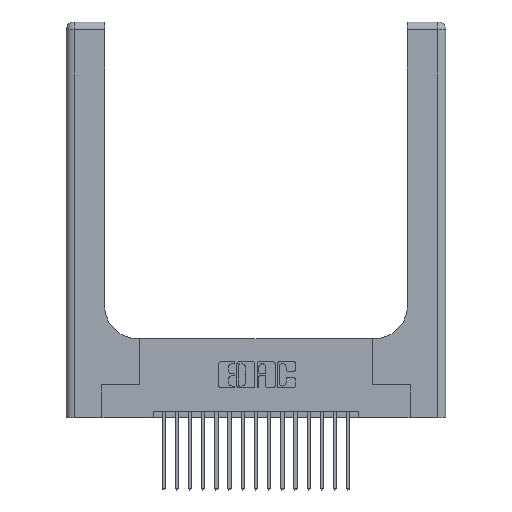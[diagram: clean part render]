
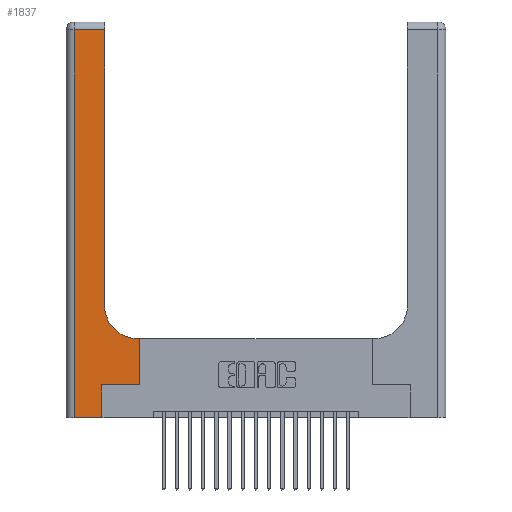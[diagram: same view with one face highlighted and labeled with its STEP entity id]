
A CAD part, top view. The second image highlights one B-rep face of the part: STEP entity #1837.
In plain terms, the highlighted planar face has unit normal (0, 0, 1).
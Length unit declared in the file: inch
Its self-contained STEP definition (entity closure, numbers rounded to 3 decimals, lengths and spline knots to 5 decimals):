
#257 = CARTESIAN_POINT ( 'NONE',  ( 0.2915, 0.85, 0.37 ) ) ;
#575 = CARTESIAN_POINT ( 'NONE',  ( 0.269, 0.25, 0.37 ) ) ;
#672 = EDGE_CURVE ( 'NONE', #4293, #8907, #10846, .T. ) ;
#947 = EDGE_CURVE ( 'NONE', #12683, #18652, #14806, .T. ) ;
#1517 = DIRECTION ( 'NONE',  ( 0., 1., 0. ) ) ;
#1659 = EDGE_CURVE ( 'NONE', #7958, #4293, #12326, .T. ) ;
#1776 = CARTESIAN_POINT ( 'NONE',  ( 0.5585, 0.25, 0.37 ) ) ;
#1837 = ADVANCED_FACE ( 'NONE', ( #2304 ), #4519, .F. ) ;
#2304 = FACE_OUTER_BOUND ( 'NONE', #10677, .T. ) ;
#2469 = CARTESIAN_POINT ( 'NONE',  ( 0.06, 2.94, 0.37 ) ) ;
#2592 = ORIENTED_EDGE ( 'NONE', *, *, #672, .T. ) ;
#2725 = AXIS2_PLACEMENT_3D ( 'NONE', #3398, #16216, #9618 ) ;
#2793 = VECTOR ( 'NONE', #1517, 39.37008 ) ;
#3398 = CARTESIAN_POINT ( 'NONE',  ( 0.5415, 0.85, 0.37 ) ) ;
#4293 = VERTEX_POINT ( 'NONE', #8136 ) ;
#4519 = PLANE ( 'NONE',  #13219 ) ;
#4549 = VECTOR ( 'NONE', #8510, 39.37008 ) ;
#4585 = DIRECTION ( 'NONE',  ( 0., 0., -1. ) ) ;
#5296 = DIRECTION ( 'NONE',  ( 1., 0., 0. ) ) ;
#5418 = LINE ( 'NONE', #10536, #17626 ) ;
#5809 = VECTOR ( 'NONE', #12511, 39.37008 ) ;
#5969 = DIRECTION ( 'NONE',  ( 0., 1., 0. ) ) ;
#6001 = VERTEX_POINT ( 'NONE', #10919 ) ;
#6007 = DIRECTION ( 'NONE',  ( -1., 0., 0. ) ) ;
#6069 = CARTESIAN_POINT ( 'NONE',  ( 0., 3., 0.37 ) ) ;
#6284 = DIRECTION ( 'NONE',  ( -1., 0., 0. ) ) ;
#6360 = ORIENTED_EDGE ( 'NONE', *, *, #1659, .T. ) ;
#6501 = ORIENTED_EDGE ( 'NONE', *, *, #14328, .T. ) ;
#7059 = EDGE_CURVE ( 'NONE', #18652, #7958, #15756, .T. ) ;
#7414 = CARTESIAN_POINT ( 'NONE',  ( 0.269, 0., 0.37 ) ) ;
#7958 = VERTEX_POINT ( 'NONE', #1776 ) ;
#8136 = CARTESIAN_POINT ( 'NONE',  ( 0.5585, 0.6, 0.37 ) ) ;
#8423 = EDGE_CURVE ( 'NONE', #6001, #12683, #16454, .T. ) ;
#8510 = DIRECTION ( 'NONE',  ( 0., 1., 0. ) ) ;
#8810 = ORIENTED_EDGE ( 'NONE', *, *, #10889, .T. ) ;
#8815 = EDGE_CURVE ( 'NONE', #9017, #10373, #9717, .T. ) ;
#8907 = VERTEX_POINT ( 'NONE', #17995 ) ;
#9017 = VERTEX_POINT ( 'NONE', #13643 ) ;
#9618 = DIRECTION ( 'NONE',  ( 1., 0., 0. ) ) ;
#9652 = ORIENTED_EDGE ( 'NONE', *, *, #8423, .T. ) ;
#9717 = LINE ( 'NONE', #11124, #15937 ) ;
#10373 = VERTEX_POINT ( 'NONE', #2469 ) ;
#10536 = CARTESIAN_POINT ( 'NONE',  ( 0.2915, 3., 0.37 ) ) ;
#10677 = EDGE_LOOP ( 'NONE', ( #12181, #19036, #6501, #9652, #14218, #12870, #6360, #2592, #8810 ) ) ;
#10846 = LINE ( 'NONE', #11133, #16059 ) ;
#10889 = EDGE_CURVE ( 'NONE', #8907, #17155, #17825, .T. ) ;
#10919 = CARTESIAN_POINT ( 'NONE',  ( 0.06, 0., 0.37 ) ) ;
#11124 = CARTESIAN_POINT ( 'NONE',  ( 0., 2.94, 0.37 ) ) ;
#11133 = CARTESIAN_POINT ( 'NONE',  ( 0.2915, 0.6, 0.37 ) ) ;
#11276 = CARTESIAN_POINT ( 'NONE',  ( 0.269, 0., 0.37 ) ) ;
#11545 = VECTOR ( 'NONE', #5296, 39.37008 ) ;
#12181 = ORIENTED_EDGE ( 'NONE', *, *, #13253, .T. ) ;
#12274 = VECTOR ( 'NONE', #16063, 39.37008 ) ;
#12326 = LINE ( 'NONE', #12909, #2793 ) ;
#12511 = DIRECTION ( 'NONE',  ( 0., -1., 0. ) ) ;
#12683 = VERTEX_POINT ( 'NONE', #7414 ) ;
#12836 = CARTESIAN_POINT ( 'NONE',  ( 0., 0., 0.37 ) ) ;
#12870 = ORIENTED_EDGE ( 'NONE', *, *, #7059, .T. ) ;
#12909 = CARTESIAN_POINT ( 'NONE',  ( 0.5585, 0.25, 0.37 ) ) ;
#13219 = AXIS2_PLACEMENT_3D ( 'NONE', #6069, #4585, #6007 ) ;
#13253 = EDGE_CURVE ( 'NONE', #17155, #9017, #5418, .T. ) ;
#13643 = CARTESIAN_POINT ( 'NONE',  ( 0.2915, 2.94, 0.37 ) ) ;
#14218 = ORIENTED_EDGE ( 'NONE', *, *, #947, .T. ) ;
#14328 = EDGE_CURVE ( 'NONE', #10373, #6001, #18724, .T. ) ;
#14445 = DIRECTION ( 'NONE',  ( -1., 0., 0. ) ) ;
#14806 = LINE ( 'NONE', #11276, #4549 ) ;
#14877 = CARTESIAN_POINT ( 'NONE',  ( 0.269, 0.25, 0.37 ) ) ;
#15756 = LINE ( 'NONE', #14877, #11545 ) ;
#15937 = VECTOR ( 'NONE', #14445, 39.37008 ) ;
#16059 = VECTOR ( 'NONE', #6284, 39.37008 ) ;
#16063 = DIRECTION ( 'NONE',  ( 1., 0., 0. ) ) ;
#16216 = DIRECTION ( 'NONE',  ( 0., 0., -1. ) ) ;
#16454 = LINE ( 'NONE', #12836, #12274 ) ;
#17155 = VERTEX_POINT ( 'NONE', #257 ) ;
#17371 = CARTESIAN_POINT ( 'NONE',  ( 0.06, 3., 0.37 ) ) ;
#17626 = VECTOR ( 'NONE', #5969, 39.37008 ) ;
#17825 = CIRCLE ( 'NONE', #2725, 0.25 ) ;
#17995 = CARTESIAN_POINT ( 'NONE',  ( 0.5415, 0.6, 0.37 ) ) ;
#18652 = VERTEX_POINT ( 'NONE', #575 ) ;
#18724 = LINE ( 'NONE', #17371, #5809 ) ;
#19036 = ORIENTED_EDGE ( 'NONE', *, *, #8815, .T. ) ;
